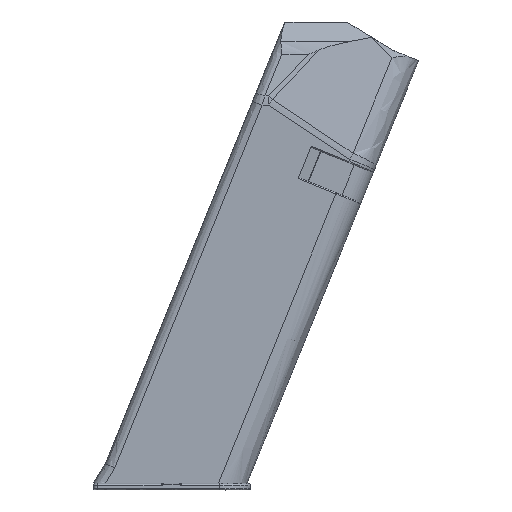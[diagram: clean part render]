
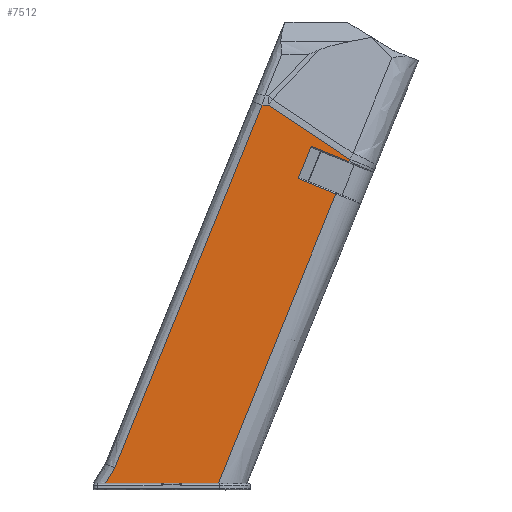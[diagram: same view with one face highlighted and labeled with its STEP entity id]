
A CAD part, top view. The second image highlights one B-rep face of the part: STEP entity #7512.
In plain terms, the highlighted planar face has unit normal (0, 0, 1).
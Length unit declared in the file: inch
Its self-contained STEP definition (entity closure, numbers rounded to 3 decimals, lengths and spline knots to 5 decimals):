
#619=PLANE('',#8084);
#1012=LINE('',#10091,#1685);
#1616=LINE('',#13616,#2289);
#1617=LINE('',#13666,#2290);
#1618=LINE('',#13669,#2291);
#1619=LINE('',#13671,#2292);
#1620=LINE('',#13673,#2293);
#1621=LINE('',#13675,#2294);
#1622=LINE('',#13677,#2295);
#1623=LINE('',#13679,#2296);
#1624=LINE('',#13680,#2297);
#1685=VECTOR('',#8204,38.6707);
#2289=VECTOR('',#9700,0.3937);
#2290=VECTOR('',#9705,0.3937);
#2291=VECTOR('',#9708,40.55118);
#2292=VECTOR('',#9709,38.38583);
#2293=VECTOR('',#9710,40.55118);
#2294=VECTOR('',#9711,38.46707);
#2295=VECTOR('',#9712,38.6707);
#2296=VECTOR('',#9713,40.55118);
#2297=VECTOR('',#9714,40.48904);
#2697=FACE_OUTER_BOUND('',#3099,.T.);
#3099=EDGE_LOOP('',(#6747,#6748,#6749,#6750,#6751,#6752,#6753,#6754,#6755,
#6756));
#3352=VERTEX_POINT('',#10088);
#3353=VERTEX_POINT('',#10090);
#3947=VERTEX_POINT('',#13609);
#3950=VERTEX_POINT('',#13614);
#3952=VERTEX_POINT('',#13668);
#3953=VERTEX_POINT('',#13670);
#3954=VERTEX_POINT('',#13672);
#3955=VERTEX_POINT('',#13674);
#3956=VERTEX_POINT('',#13676);
#3957=VERTEX_POINT('',#13678);
#4018=EDGE_CURVE('',#3352,#3353,#1012,.T.);
#4923=EDGE_CURVE('',#3950,#3947,#1616,.T.);
#4927=EDGE_CURVE('',#3352,#3947,#1617,.T.);
#4928=EDGE_CURVE('',#3952,#3950,#1618,.T.);
#4929=EDGE_CURVE('',#3952,#3953,#1619,.T.);
#4930=EDGE_CURVE('',#3953,#3954,#1620,.T.);
#4931=EDGE_CURVE('',#3954,#3955,#1621,.T.);
#4932=EDGE_CURVE('',#3955,#3956,#1622,.T.);
#4933=EDGE_CURVE('',#3956,#3957,#1623,.T.);
#4934=EDGE_CURVE('',#3957,#3353,#1624,.T.);
#6747=ORIENTED_EDGE('',*,*,#4018,.F.);
#6748=ORIENTED_EDGE('',*,*,#4927,.T.);
#6749=ORIENTED_EDGE('',*,*,#4923,.F.);
#6750=ORIENTED_EDGE('',*,*,#4928,.F.);
#6751=ORIENTED_EDGE('',*,*,#4929,.T.);
#6752=ORIENTED_EDGE('',*,*,#4930,.T.);
#6753=ORIENTED_EDGE('',*,*,#4931,.T.);
#6754=ORIENTED_EDGE('',*,*,#4932,.T.);
#6755=ORIENTED_EDGE('',*,*,#4933,.T.);
#6756=ORIENTED_EDGE('',*,*,#4934,.T.);
#7512=ADVANCED_FACE('',(#2697),#619,.T.);
#8084=AXIS2_PLACEMENT_3D('',#13667,#9706,#9707);
#8204=DIRECTION('',(-1.,0.,0.));
#9700=DIRECTION('',(0.927,-0.376,0.));
#9705=DIRECTION('',(0.376,0.927,0.));
#9706=DIRECTION('center_axis',(0.,0.,1.));
#9707=DIRECTION('ref_axis',(0.927,-0.376,0.));
#9708=DIRECTION('',(-0.376,-0.927,0.));
#9709=DIRECTION('',(0.927,-0.376,0.));
#9710=DIRECTION('',(0.376,0.927,0.));
#9711=DIRECTION('',(-0.832,0.555,0.));
#9712=DIRECTION('',(-1.,0.,0.));
#9713=DIRECTION('',(-0.376,-0.927,0.));
#9714=DIRECTION('',(-0.522,-0.853,0.));
#10088=CARTESIAN_POINT('',(1.78225,-0.0556,0.45379));
#10090=CARTESIAN_POINT('',(0.71713,-0.0551,0.45379));
#10091=CARTESIAN_POINT('',(0.70528,-0.0551,0.45379));
#13609=CARTESIAN_POINT('',(2.88897,2.66991,0.45379));
#13614=CARTESIAN_POINT('',(2.53331,2.81433,0.45379));
#13616=CARTESIAN_POINT('',(2.92608,2.65484,0.45379));
#13666=CARTESIAN_POINT('',(2.88671,2.66435,0.45379));
#13667=CARTESIAN_POINT('Origin',(3.00039,2.61272,0.45379));
#13668=CARTESIAN_POINT('',(2.65692,3.11874,0.45379));
#13669=CARTESIAN_POINT('',(2.6531,3.10934,0.45379));
#13670=CARTESIAN_POINT('',(3.01257,2.97432,0.45379));
#13671=CARTESIAN_POINT('',(2.08787,3.3498,0.45379));
#13672=CARTESIAN_POINT('',(3.02094,2.99493,0.45379));
#13673=CARTESIAN_POINT('',(3.00163,2.94738,0.45379));
#13674=CARTESIAN_POINT('',(2.2546,3.50648,0.45379));
#13675=CARTESIAN_POINT('',(3.17963,2.88901,0.45379));
#13676=CARTESIAN_POINT('',(2.19293,3.5065,0.45379));
#13677=CARTESIAN_POINT('',(0.8378,3.50713,0.45379));
#13678=CARTESIAN_POINT('',(0.80505,0.08856,0.45379));
#13679=CARTESIAN_POINT('',(0.80834,0.09669,0.45379));
#13680=CARTESIAN_POINT('',(0.79286,0.06864,0.45379));
